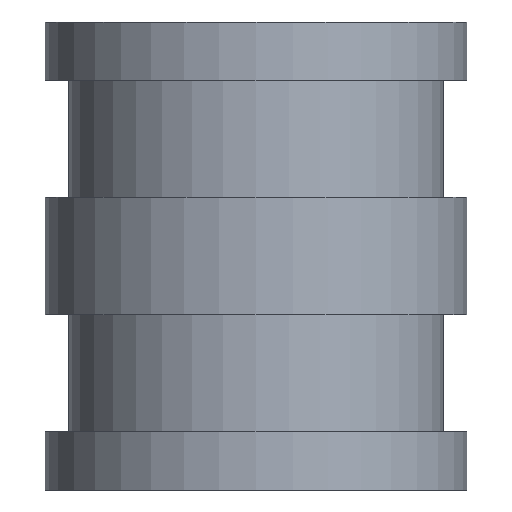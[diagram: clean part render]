
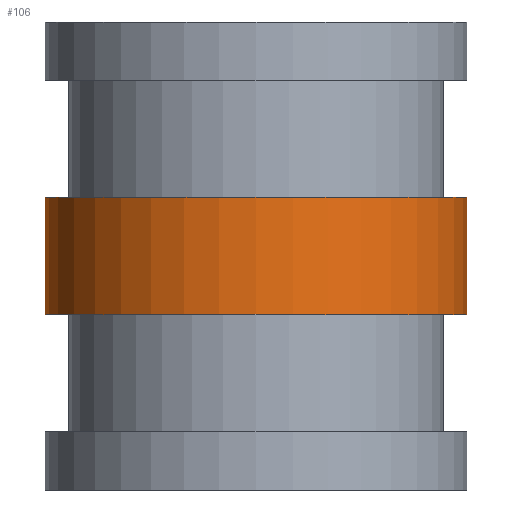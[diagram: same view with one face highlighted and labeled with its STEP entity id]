
A CAD part, front view. The second image highlights one B-rep face of the part: STEP entity #106.
In plain terms, the highlighted cylindrical face has radius 22.86 mm (diameter 45.72 mm), a partial arc.
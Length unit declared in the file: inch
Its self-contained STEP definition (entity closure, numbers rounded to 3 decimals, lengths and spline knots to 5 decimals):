
#1 = DIRECTION ( 'NONE',  ( -1., 0., 0. ) ) ;
#8 = ORIENTED_EDGE ( 'NONE', *, *, #282, .F. ) ;
#15 = AXIS2_PLACEMENT_3D ( 'NONE', #422, #188, #1 ) ;
#28 = DIRECTION ( 'NONE',  ( 0., 0., -1. ) ) ;
#81 = AXIS2_PLACEMENT_3D ( 'NONE', #100, #126, #128 ) ;
#92 = CARTESIAN_POINT ( 'NONE',  ( -0.9, 0.1607, -2.25 ) ) ;
#100 = CARTESIAN_POINT ( 'NONE',  ( 0., 0.1607, -1. ) ) ;
#106 = ADVANCED_FACE ( 'NONE', ( #459 ), #450, .T. ) ;
#126 = DIRECTION ( 'NONE',  ( 0., 0., -1. ) ) ;
#128 = DIRECTION ( 'NONE',  ( -1., 0., 0. ) ) ;
#183 = CARTESIAN_POINT ( 'NONE',  ( -0.9, 0.1607, -1.75 ) ) ;
#188 = DIRECTION ( 'NONE',  ( 0., 0., -1. ) ) ;
#209 = EDGE_CURVE ( 'NONE', #315, #477, #393, .T. ) ;
#222 = CARTESIAN_POINT ( 'NONE',  ( 0.9, 0.1607, -1. ) ) ;
#234 = EDGE_CURVE ( 'NONE', #276, #315, #388, .T. ) ;
#248 = EDGE_CURVE ( 'NONE', #276, #348, #367, .T. ) ;
#252 = ORIENTED_EDGE ( 'NONE', *, *, #234, .F. ) ;
#263 = DIRECTION ( 'NONE',  ( -1., 0., 0. ) ) ;
#267 = CARTESIAN_POINT ( 'NONE',  ( 0.9, 0.1607, -2.25 ) ) ;
#276 = VERTEX_POINT ( 'NONE', #398 ) ;
#282 = EDGE_CURVE ( 'NONE', #477, #348, #352, .T. ) ;
#303 = ORIENTED_EDGE ( 'NONE', *, *, #209, .F. ) ;
#310 = CARTESIAN_POINT ( 'NONE',  ( 0., 0.1607, -1.75 ) ) ;
#315 = VERTEX_POINT ( 'NONE', #267 ) ;
#338 = DIRECTION ( 'NONE',  ( 0., 0., 1. ) ) ;
#344 = VECTOR ( 'NONE', #338, 39.37008 ) ;
#348 = VERTEX_POINT ( 'NONE', #183 ) ;
#349 = ORIENTED_EDGE ( 'NONE', *, *, #248, .T. ) ;
#352 = LINE ( 'NONE', #403, #344 ) ;
#364 = DIRECTION ( 'NONE',  ( 0., 0., -1. ) ) ;
#367 = CIRCLE ( 'NONE', #482, 0.9 ) ;
#384 = VECTOR ( 'NONE', #364, 39.37008 ) ;
#388 = LINE ( 'NONE', #222, #384 ) ;
#393 = CIRCLE ( 'NONE', #15, 0.9 ) ;
#398 = CARTESIAN_POINT ( 'NONE',  ( 0.9, 0.1607, -1.75 ) ) ;
#403 = CARTESIAN_POINT ( 'NONE',  ( -0.9, 0.1607, -1. ) ) ;
#422 = CARTESIAN_POINT ( 'NONE',  ( 0., 0.1607, -2.25 ) ) ;
#450 = CYLINDRICAL_SURFACE ( 'NONE', #81, 0.9 ) ;
#459 = FACE_OUTER_BOUND ( 'NONE', #483, .T. ) ;
#477 = VERTEX_POINT ( 'NONE', #92 ) ;
#482 = AXIS2_PLACEMENT_3D ( 'NONE', #310, #28, #263 ) ;
#483 = EDGE_LOOP ( 'NONE', ( #252, #349, #8, #303 ) ) ;
